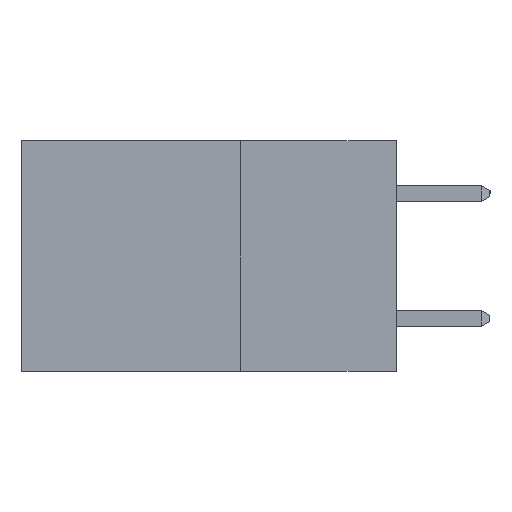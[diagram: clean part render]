
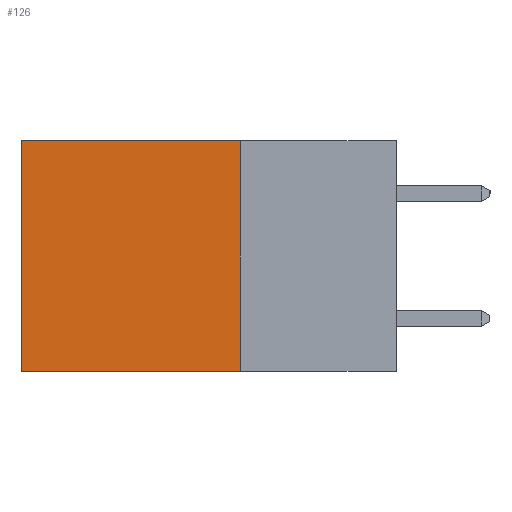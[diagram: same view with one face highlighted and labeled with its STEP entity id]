
A CAD part, left-side view. The second image highlights one B-rep face of the part: STEP entity #126.
In plain terms, the highlighted planar face has unit normal (-1, 0, 0).
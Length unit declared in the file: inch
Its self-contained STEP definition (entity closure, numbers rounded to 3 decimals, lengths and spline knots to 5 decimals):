
#5 = CARTESIAN_POINT ( 'NONE',  ( 0.2615, 0.6, 0. ) ) ;
#126 = ADVANCED_FACE ( 'NONE', ( #2889 ), #10297, .F. ) ;
#202 = ORIENTED_EDGE ( 'NONE', *, *, #9060, .T. ) ;
#392 = VECTOR ( 'NONE', #10448, 39.37008 ) ;
#544 = VECTOR ( 'NONE', #9962, 39.37008 ) ;
#981 = ORIENTED_EDGE ( 'NONE', *, *, #6437, .T. ) ;
#994 = AXIS2_PLACEMENT_3D ( 'NONE', #1946, #7070, #5331 ) ;
#1120 = ORIENTED_EDGE ( 'NONE', *, *, #7569, .F. ) ;
#1419 = VERTEX_POINT ( 'NONE', #5380 ) ;
#1425 = CARTESIAN_POINT ( 'NONE',  ( 0.2615, 0.25, -0.37 ) ) ;
#1946 = CARTESIAN_POINT ( 'NONE',  ( 0.2615, 0.25, -0.37 ) ) ;
#2889 = FACE_OUTER_BOUND ( 'NONE', #10372, .T. ) ;
#3413 = VERTEX_POINT ( 'NONE', #1425 ) ;
#3655 = LINE ( 'NONE', #8795, #10140 ) ;
#4285 = CARTESIAN_POINT ( 'NONE',  ( 0.2615, 0.25, 0. ) ) ;
#4730 = VERTEX_POINT ( 'NONE', #5 ) ;
#5331 = DIRECTION ( 'NONE',  ( 0., 0., -1. ) ) ;
#5362 = ORIENTED_EDGE ( 'NONE', *, *, #7165, .F. ) ;
#5380 = CARTESIAN_POINT ( 'NONE',  ( 0.2615, 0.6, -0.37 ) ) ;
#5548 = LINE ( 'NONE', #7837, #392 ) ;
#6201 = VECTOR ( 'NONE', #9971, 39.37008 ) ;
#6317 = DIRECTION ( 'NONE',  ( 0., 0., -1. ) ) ;
#6437 = EDGE_CURVE ( 'NONE', #4730, #1419, #3655, .T. ) ;
#7070 = DIRECTION ( 'NONE',  ( 1., 0., 0. ) ) ;
#7165 = EDGE_CURVE ( 'NONE', #7577, #3413, #9401, .T. ) ;
#7569 = EDGE_CURVE ( 'NONE', #3413, #1419, #8310, .T. ) ;
#7577 = VERTEX_POINT ( 'NONE', #4285 ) ;
#7837 = CARTESIAN_POINT ( 'NONE',  ( 0.2615, 0.25, 0. ) ) ;
#8310 = LINE ( 'NONE', #9338, #544 ) ;
#8795 = CARTESIAN_POINT ( 'NONE',  ( 0.2615, 0.6, -0.37 ) ) ;
#9060 = EDGE_CURVE ( 'NONE', #7577, #4730, #5548, .T. ) ;
#9338 = CARTESIAN_POINT ( 'NONE',  ( 0.2615, 0.25, -0.37 ) ) ;
#9401 = LINE ( 'NONE', #10199, #6201 ) ;
#9962 = DIRECTION ( 'NONE',  ( 0., 1., 0. ) ) ;
#9971 = DIRECTION ( 'NONE',  ( 0., 0., -1. ) ) ;
#10140 = VECTOR ( 'NONE', #6317, 39.37008 ) ;
#10199 = CARTESIAN_POINT ( 'NONE',  ( 0.2615, 0.25, -0.37 ) ) ;
#10297 = PLANE ( 'NONE',  #994 ) ;
#10372 = EDGE_LOOP ( 'NONE', ( #981, #1120, #5362, #202 ) ) ;
#10448 = DIRECTION ( 'NONE',  ( 0., 1., 0. ) ) ;
